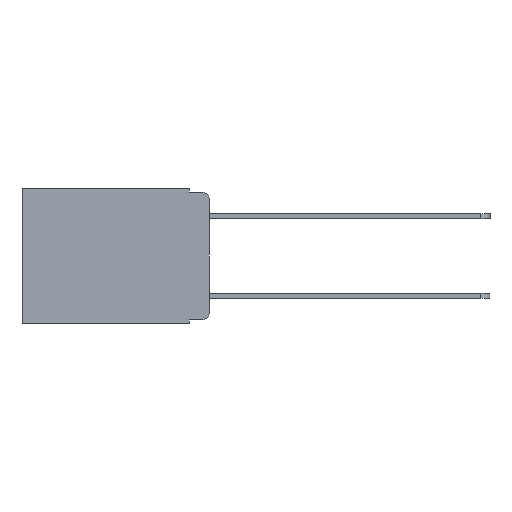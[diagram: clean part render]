
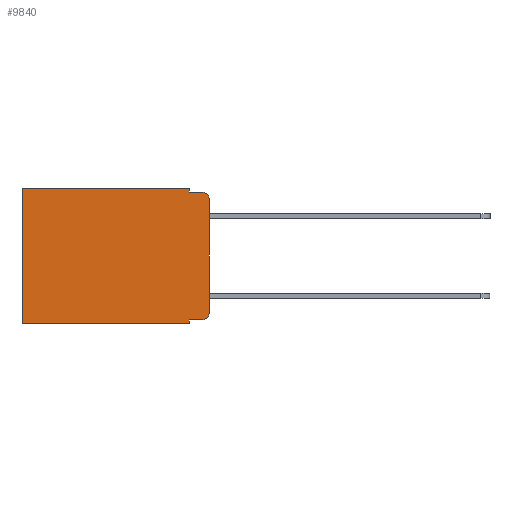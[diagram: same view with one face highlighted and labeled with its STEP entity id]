
A CAD part, left-side view. The second image highlights one B-rep face of the part: STEP entity #9840.
In plain terms, the highlighted planar face has unit normal (-1, 0, 0).
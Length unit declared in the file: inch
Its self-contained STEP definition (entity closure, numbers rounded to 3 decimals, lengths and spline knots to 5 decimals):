
#23 = DIRECTION ( 'NONE',  ( -1., 0., 0. ) ) ;
#314 = AXIS2_PLACEMENT_3D ( 'NONE', #5351, #23, #6175 ) ;
#323 = CARTESIAN_POINT ( 'NONE',  ( 0.298, 0.02, -0.313 ) ) ;
#351 = VECTOR ( 'NONE', #6653, 39.37008 ) ;
#759 = EDGE_CURVE ( 'NONE', #9456, #11040, #5995, .T. ) ;
#829 = DIRECTION ( 'NONE',  ( 0., 0., -1. ) ) ;
#1033 = VERTEX_POINT ( 'NONE', #5159 ) ;
#1240 = ORIENTED_EDGE ( 'NONE', *, *, #4546, .T. ) ;
#1394 = CARTESIAN_POINT ( 'NONE',  ( 0.298, 0.473, -0.343 ) ) ;
#1398 = CARTESIAN_POINT ( 'NONE',  ( 0.298, 0.051, -0.333 ) ) ;
#1411 = EDGE_CURVE ( 'NONE', #11064, #9456, #5086, .T. ) ;
#1428 = LINE ( 'NONE', #8892, #3548 ) ;
#1580 = VECTOR ( 'NONE', #10201, 39.37008 ) ;
#1667 = DIRECTION ( 'NONE',  ( 0., 1., 0. ) ) ;
#1807 = ORIENTED_EDGE ( 'NONE', *, *, #3217, .F. ) ;
#1856 = LINE ( 'NONE', #8562, #6355 ) ;
#1975 = CARTESIAN_POINT ( 'NONE',  ( 0.298, 0.051, -0.333 ) ) ;
#2012 = EDGE_CURVE ( 'NONE', #11064, #2306, #1428, .T. ) ;
#2022 = EDGE_LOOP ( 'NONE', ( #8007, #1240, #6056, #1807, #6573, #2095, #6835, #11275, #2388, #5174 ) ) ;
#2053 = VECTOR ( 'NONE', #3727, 39.37008 ) ;
#2095 = ORIENTED_EDGE ( 'NONE', *, *, #2597, .T. ) ;
#2173 = CIRCLE ( 'NONE', #314, 0.02 ) ;
#2223 = VERTEX_POINT ( 'NONE', #10350 ) ;
#2306 = VERTEX_POINT ( 'NONE', #6951 ) ;
#2388 = ORIENTED_EDGE ( 'NONE', *, *, #1411, .T. ) ;
#2389 = LINE ( 'NONE', #9553, #6837 ) ;
#2597 = EDGE_CURVE ( 'NONE', #7155, #6483, #6350, .T. ) ;
#2925 = CARTESIAN_POINT ( 'NONE',  ( 0.298, 0.051, -0.01 ) ) ;
#3104 = FACE_OUTER_BOUND ( 'NONE', #2022, .T. ) ;
#3201 = LINE ( 'NONE', #4878, #5405 ) ;
#3217 = EDGE_CURVE ( 'NONE', #2223, #6296, #3201, .T. ) ;
#3529 = DIRECTION ( 'NONE',  ( 0., 0., -1. ) ) ;
#3548 = VECTOR ( 'NONE', #8658, 39.37008 ) ;
#3559 = PLANE ( 'NONE',  #5509 ) ;
#3727 = DIRECTION ( 'NONE',  ( 0., -1., 0. ) ) ;
#3846 = DIRECTION ( 'NONE',  ( 0., 0., -1. ) ) ;
#3870 = EDGE_CURVE ( 'NONE', #6296, #1033, #4859, .T. ) ;
#4330 = DIRECTION ( 'NONE',  ( 0., 1., 0. ) ) ;
#4546 = EDGE_CURVE ( 'NONE', #8038, #1033, #2173, .T. ) ;
#4859 = LINE ( 'NONE', #2925, #2053 ) ;
#4878 = CARTESIAN_POINT ( 'NONE',  ( 0.298, 0.051, 0. ) ) ;
#5086 = LINE ( 'NONE', #1398, #351 ) ;
#5159 = CARTESIAN_POINT ( 'NONE',  ( 0.298, 0.02, -0.01 ) ) ;
#5174 = ORIENTED_EDGE ( 'NONE', *, *, #759, .T. ) ;
#5351 = CARTESIAN_POINT ( 'NONE',  ( 0.298, 0.02, -0.03 ) ) ;
#5405 = VECTOR ( 'NONE', #3529, 39.37008 ) ;
#5443 = CARTESIAN_POINT ( 'NONE',  ( 0.298, 0., 0. ) ) ;
#5492 = EDGE_CURVE ( 'NONE', #2306, #6483, #1856, .T. ) ;
#5509 = AXIS2_PLACEMENT_3D ( 'NONE', #5443, #6264, #829 ) ;
#5706 = EDGE_CURVE ( 'NONE', #8038, #11040, #5855, .T. ) ;
#5851 = CARTESIAN_POINT ( 'NONE',  ( 0.298, 0.02, -0.333 ) ) ;
#5855 = LINE ( 'NONE', #6084, #7662 ) ;
#5995 = CIRCLE ( 'NONE', #7712, 0.02 ) ;
#6056 = ORIENTED_EDGE ( 'NONE', *, *, #3870, .F. ) ;
#6084 = CARTESIAN_POINT ( 'NONE',  ( 0.298, 0., 0. ) ) ;
#6175 = DIRECTION ( 'NONE',  ( 0., 0., -1. ) ) ;
#6264 = DIRECTION ( 'NONE',  ( 1., 0., 0. ) ) ;
#6296 = VERTEX_POINT ( 'NONE', #10286 ) ;
#6350 = LINE ( 'NONE', #9805, #1580 ) ;
#6355 = VECTOR ( 'NONE', #4330, 39.37008 ) ;
#6483 = VERTEX_POINT ( 'NONE', #1394 ) ;
#6573 = ORIENTED_EDGE ( 'NONE', *, *, #10884, .T. ) ;
#6653 = DIRECTION ( 'NONE',  ( 0., -1., 0. ) ) ;
#6835 = ORIENTED_EDGE ( 'NONE', *, *, #5492, .F. ) ;
#6837 = VECTOR ( 'NONE', #1667, 39.37008 ) ;
#6921 = DIRECTION ( 'NONE',  ( 0., 0., -1. ) ) ;
#6951 = CARTESIAN_POINT ( 'NONE',  ( 0.298, 0.051, -0.343 ) ) ;
#7155 = VERTEX_POINT ( 'NONE', #7727 ) ;
#7246 = CARTESIAN_POINT ( 'NONE',  ( 0.298, 0., -0.313 ) ) ;
#7662 = VECTOR ( 'NONE', #6921, 39.37008 ) ;
#7712 = AXIS2_PLACEMENT_3D ( 'NONE', #323, #7955, #3846 ) ;
#7727 = CARTESIAN_POINT ( 'NONE',  ( 0.298, 0.473, 0. ) ) ;
#7955 = DIRECTION ( 'NONE',  ( -1., 0., 0. ) ) ;
#8007 = ORIENTED_EDGE ( 'NONE', *, *, #5706, .F. ) ;
#8038 = VERTEX_POINT ( 'NONE', #9758 ) ;
#8562 = CARTESIAN_POINT ( 'NONE',  ( 0.298, 0., -0.343 ) ) ;
#8658 = DIRECTION ( 'NONE',  ( 0., 0., -1. ) ) ;
#8892 = CARTESIAN_POINT ( 'NONE',  ( 0.298, 0.051, 0. ) ) ;
#9456 = VERTEX_POINT ( 'NONE', #5851 ) ;
#9553 = CARTESIAN_POINT ( 'NONE',  ( 0.298, 0., 0. ) ) ;
#9758 = CARTESIAN_POINT ( 'NONE',  ( 0.298, 0., -0.03 ) ) ;
#9805 = CARTESIAN_POINT ( 'NONE',  ( 0.298, 0.473, 0. ) ) ;
#9840 = ADVANCED_FACE ( 'NONE', ( #3104 ), #3559, .F. ) ;
#10201 = DIRECTION ( 'NONE',  ( 0., 0., -1. ) ) ;
#10286 = CARTESIAN_POINT ( 'NONE',  ( 0.298, 0.051, -0.01 ) ) ;
#10350 = CARTESIAN_POINT ( 'NONE',  ( 0.298, 0.051, 0. ) ) ;
#10884 = EDGE_CURVE ( 'NONE', #2223, #7155, #2389, .T. ) ;
#11040 = VERTEX_POINT ( 'NONE', #7246 ) ;
#11064 = VERTEX_POINT ( 'NONE', #1975 ) ;
#11275 = ORIENTED_EDGE ( 'NONE', *, *, #2012, .F. ) ;
